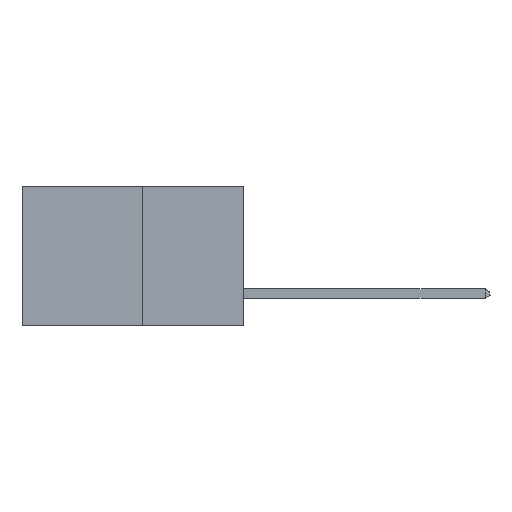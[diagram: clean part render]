
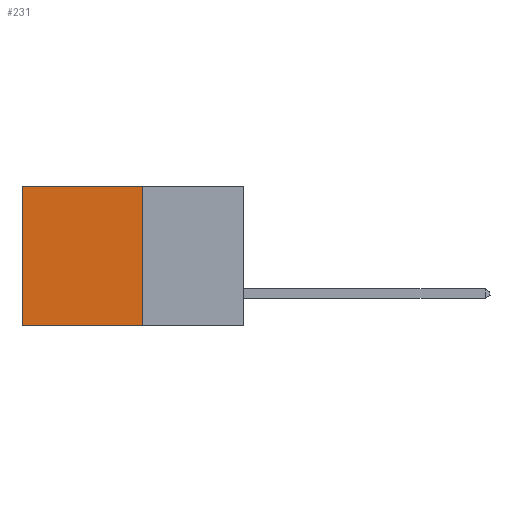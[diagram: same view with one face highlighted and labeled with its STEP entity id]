
A CAD part, left-side view. The second image highlights one B-rep face of the part: STEP entity #231.
In plain terms, the highlighted planar face has unit normal (-1, 0, 0).
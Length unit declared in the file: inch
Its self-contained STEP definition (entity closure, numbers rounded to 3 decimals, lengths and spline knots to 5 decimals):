
#231 = ADVANCED_FACE ( 'NONE', ( #6622 ), #6083, .F. ) ;
#778 = DIRECTION ( 'NONE',  ( 0., 0., -1. ) ) ;
#793 = DIRECTION ( 'NONE',  ( 1., 0., 0. ) ) ;
#839 = CARTESIAN_POINT ( 'NONE',  ( 0.277, 0.27, -0.37 ) ) ;
#1080 = VECTOR ( 'NONE', #8484, 39.37008 ) ;
#1667 = VERTEX_POINT ( 'NONE', #10825 ) ;
#1944 = DIRECTION ( 'NONE',  ( 0., 1., 0. ) ) ;
#2470 = ORIENTED_EDGE ( 'NONE', *, *, #4074, .F. ) ;
#2765 = ORIENTED_EDGE ( 'NONE', *, *, #5292, .T. ) ;
#3002 = VECTOR ( 'NONE', #14737, 39.37008 ) ;
#3549 = ORIENTED_EDGE ( 'NONE', *, *, #7168, .T. ) ;
#4074 = EDGE_CURVE ( 'NONE', #12955, #1667, #13533, .T. ) ;
#5004 = LINE ( 'NONE', #8658, #13781 ) ;
#5292 = EDGE_CURVE ( 'NONE', #7063, #9628, #15226, .T. ) ;
#6083 = PLANE ( 'NONE',  #8704 ) ;
#6622 = FACE_OUTER_BOUND ( 'NONE', #8868, .T. ) ;
#7063 = VERTEX_POINT ( 'NONE', #12024 ) ;
#7168 = EDGE_CURVE ( 'NONE', #12955, #7063, #5004, .T. ) ;
#8050 = CARTESIAN_POINT ( 'NONE',  ( 0.277, 0.27, -0.37 ) ) ;
#8331 = ORIENTED_EDGE ( 'NONE', *, *, #8338, .F. ) ;
#8338 = EDGE_CURVE ( 'NONE', #1667, #9628, #13571, .T. ) ;
#8484 = DIRECTION ( 'NONE',  ( 0., 0., -1. ) ) ;
#8499 = CARTESIAN_POINT ( 'NONE',  ( 0.277, 0.27, -0.37 ) ) ;
#8658 = CARTESIAN_POINT ( 'NONE',  ( 0.277, 0.27, 0. ) ) ;
#8704 = AXIS2_PLACEMENT_3D ( 'NONE', #839, #793, #778 ) ;
#8868 = EDGE_LOOP ( 'NONE', ( #2765, #8331, #2470, #3549 ) ) ;
#8976 = CARTESIAN_POINT ( 'NONE',  ( 0.277, 0.59, -0.37 ) ) ;
#9628 = VERTEX_POINT ( 'NONE', #11570 ) ;
#9886 = DIRECTION ( 'NONE',  ( 0., 1., 0. ) ) ;
#10515 = VECTOR ( 'NONE', #1944, 39.37008 ) ;
#10825 = CARTESIAN_POINT ( 'NONE',  ( 0.277, 0.27, -0.37 ) ) ;
#11570 = CARTESIAN_POINT ( 'NONE',  ( 0.277, 0.59, -0.37 ) ) ;
#12024 = CARTESIAN_POINT ( 'NONE',  ( 0.277, 0.59, 0. ) ) ;
#12955 = VERTEX_POINT ( 'NONE', #14857 ) ;
#13533 = LINE ( 'NONE', #8499, #1080 ) ;
#13571 = LINE ( 'NONE', #8050, #10515 ) ;
#13781 = VECTOR ( 'NONE', #9886, 39.37008 ) ;
#14737 = DIRECTION ( 'NONE',  ( 0., 0., -1. ) ) ;
#14857 = CARTESIAN_POINT ( 'NONE',  ( 0.277, 0.27, 0. ) ) ;
#15226 = LINE ( 'NONE', #8976, #3002 ) ;
